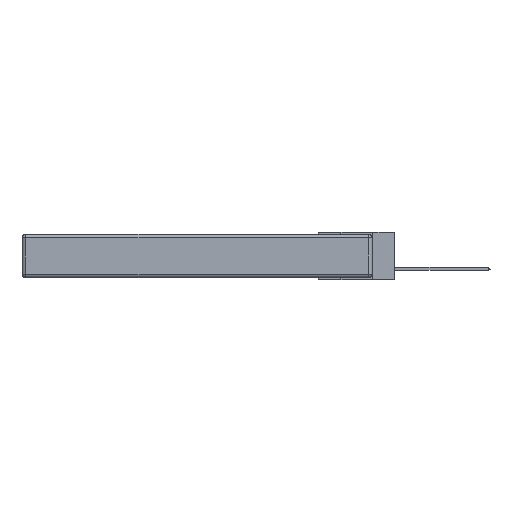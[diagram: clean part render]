
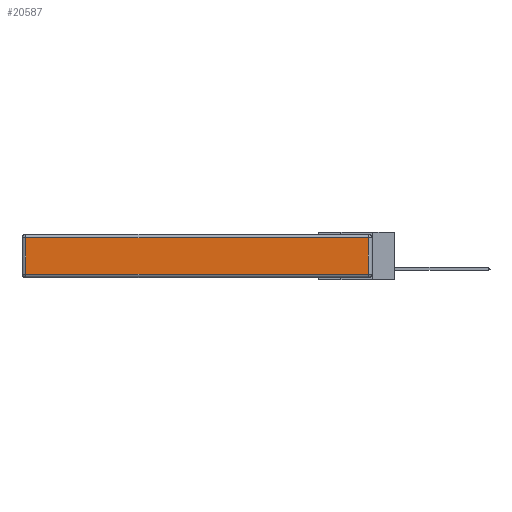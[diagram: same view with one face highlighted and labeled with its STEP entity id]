
A CAD part, left-side view. The second image highlights one B-rep face of the part: STEP entity #20587.
In plain terms, the highlighted planar face has unit normal (-1, 0, 0).
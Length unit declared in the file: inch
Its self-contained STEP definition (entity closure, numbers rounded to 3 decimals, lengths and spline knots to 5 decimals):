
#452 = LINE ( 'NONE', #25861, #24794 ) ;
#5779 = CARTESIAN_POINT ( 'NONE',  ( 0., 2.75, -0.03 ) ) ;
#8063 = CARTESIAN_POINT ( 'NONE',  ( 0., 0., -0.343 ) ) ;
#8421 = EDGE_CURVE ( 'NONE', #32085, #32333, #26177, .T. ) ;
#8708 = VECTOR ( 'NONE', #23588, 39.37008 ) ;
#9149 = ORIENTED_EDGE ( 'NONE', *, *, #28688, .T. ) ;
#9160 = ORIENTED_EDGE ( 'NONE', *, *, #8421, .T. ) ;
#10319 = ORIENTED_EDGE ( 'NONE', *, *, #25529, .T. ) ;
#10981 = CARTESIAN_POINT ( 'NONE',  ( 0., 2.72, -0.313 ) ) ;
#11078 = CARTESIAN_POINT ( 'NONE',  ( 0., 2.72, -0.343 ) ) ;
#12274 = CARTESIAN_POINT ( 'NONE',  ( 0., 2.72, -0.03 ) ) ;
#16755 = EDGE_CURVE ( 'NONE', #30852, #24446, #452, .T. ) ;
#17580 = LINE ( 'NONE', #27160, #17959 ) ;
#17959 = VECTOR ( 'NONE', #31895, 39.37008 ) ;
#18336 = ORIENTED_EDGE ( 'NONE', *, *, #16755, .T. ) ;
#18709 = CARTESIAN_POINT ( 'NONE',  ( 0., 0.03, -0.313 ) ) ;
#19445 = VECTOR ( 'NONE', #31779, 39.37008 ) ;
#20587 = ADVANCED_FACE ( 'NONE', ( #30348 ), #30719, .T. ) ;
#20649 = DIRECTION ( 'NONE',  ( 0., 0., 1. ) ) ;
#23396 = LINE ( 'NONE', #5779, #8708 ) ;
#23588 = DIRECTION ( 'NONE',  ( 0., 1., 0. ) ) ;
#24446 = VERTEX_POINT ( 'NONE', #32212 ) ;
#24794 = VECTOR ( 'NONE', #20649, 39.37008 ) ;
#25529 = EDGE_CURVE ( 'NONE', #32333, #30852, #17580, .T. ) ;
#25861 = CARTESIAN_POINT ( 'NONE',  ( 0., 0.03, -0.343 ) ) ;
#26177 = LINE ( 'NONE', #11078, #19445 ) ;
#27160 = CARTESIAN_POINT ( 'NONE',  ( 0., 0., -0.313 ) ) ;
#28688 = EDGE_CURVE ( 'NONE', #24446, #32085, #23396, .T. ) ;
#29994 = EDGE_LOOP ( 'NONE', ( #10319, #18336, #9149, #9160 ) ) ;
#30348 = FACE_OUTER_BOUND ( 'NONE', #29994, .T. ) ;
#30717 = AXIS2_PLACEMENT_3D ( 'NONE', #8063, #30936, #31033 ) ;
#30719 = PLANE ( 'NONE',  #30717 ) ;
#30852 = VERTEX_POINT ( 'NONE', #18709 ) ;
#30936 = DIRECTION ( 'NONE',  ( -1., 0., 0. ) ) ;
#31033 = DIRECTION ( 'NONE',  ( 0., 0., 1. ) ) ;
#31779 = DIRECTION ( 'NONE',  ( 0., 0., -1. ) ) ;
#31895 = DIRECTION ( 'NONE',  ( 0., -1., 0. ) ) ;
#32085 = VERTEX_POINT ( 'NONE', #12274 ) ;
#32212 = CARTESIAN_POINT ( 'NONE',  ( 0., 0.03, -0.03 ) ) ;
#32333 = VERTEX_POINT ( 'NONE', #10981 ) ;
